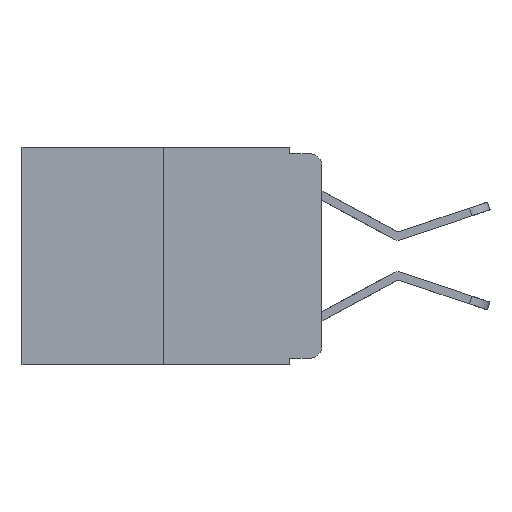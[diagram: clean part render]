
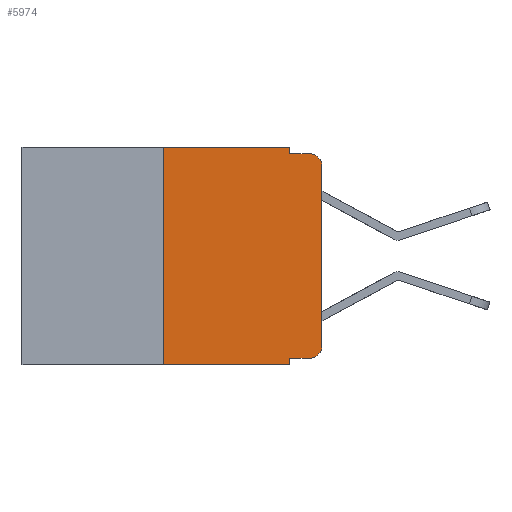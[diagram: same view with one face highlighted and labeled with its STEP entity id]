
A CAD part, left-side view. The second image highlights one B-rep face of the part: STEP entity #5974.
In plain terms, the highlighted planar face has unit normal (-1, 0, 0).
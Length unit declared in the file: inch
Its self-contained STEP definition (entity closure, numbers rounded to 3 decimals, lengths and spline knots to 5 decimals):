
#44 = CARTESIAN_POINT ( 'NONE',  ( 0., 0., 0. ) ) ;
#95 = CARTESIAN_POINT ( 'NONE',  ( 0., 0.473, 0. ) ) ;
#278 = LINE ( 'NONE', #5480, #4809 ) ;
#353 = EDGE_CURVE ( 'NONE', #7206, #18156, #7311, .T. ) ;
#650 = VERTEX_POINT ( 'NONE', #5163 ) ;
#682 = EDGE_CURVE ( 'NONE', #650, #17576, #9665, .T. ) ;
#1302 = ORIENTED_EDGE ( 'NONE', *, *, #15574, .F. ) ;
#1369 = VECTOR ( 'NONE', #10219, 39.37008 ) ;
#1646 = VECTOR ( 'NONE', #16651, 39.37008 ) ;
#2016 = ORIENTED_EDGE ( 'NONE', *, *, #12888, .T. ) ;
#2082 = EDGE_CURVE ( 'NONE', #650, #7614, #5396, .T. ) ;
#2386 = CARTESIAN_POINT ( 'NONE',  ( 0., 0.051, -0.01 ) ) ;
#2446 = CARTESIAN_POINT ( 'NONE',  ( 0., 0.02, -0.313 ) ) ;
#2654 = CARTESIAN_POINT ( 'NONE',  ( 0., 0.051, 0. ) ) ;
#2693 = LINE ( 'NONE', #13224, #3640 ) ;
#2829 = VERTEX_POINT ( 'NONE', #16984 ) ;
#2839 = EDGE_CURVE ( 'NONE', #2829, #3998, #11771, .T. ) ;
#2913 = VECTOR ( 'NONE', #13555, 39.37008 ) ;
#2977 = PLANE ( 'NONE',  #3297 ) ;
#3297 = AXIS2_PLACEMENT_3D ( 'NONE', #11960, #4524, #14995 ) ;
#3496 = CARTESIAN_POINT ( 'NONE',  ( 0., 0.051, -0.01 ) ) ;
#3525 = CARTESIAN_POINT ( 'NONE',  ( 0., 0.02, -0.03 ) ) ;
#3640 = VECTOR ( 'NONE', #4261, 39.37008 ) ;
#3788 = EDGE_LOOP ( 'NONE', ( #2016, #6495, #4403, #1302, #18246, #19176, #9107, #13548, #14967, #11889 ) ) ;
#3901 = DIRECTION ( 'NONE',  ( 0., -1., 0. ) ) ;
#3963 = DIRECTION ( 'NONE',  ( 0., 0., -1. ) ) ;
#3998 = VERTEX_POINT ( 'NONE', #14030 ) ;
#4228 = CARTESIAN_POINT ( 'NONE',  ( 0., 0.051, -0.333 ) ) ;
#4261 = DIRECTION ( 'NONE',  ( 0., 0., 1. ) ) ;
#4403 = ORIENTED_EDGE ( 'NONE', *, *, #15913, .F. ) ;
#4524 = DIRECTION ( 'NONE',  ( 1., 0., 0. ) ) ;
#4539 = CARTESIAN_POINT ( 'NONE',  ( 0., 0.25, 0. ) ) ;
#4809 = VECTOR ( 'NONE', #3901, 39.37008 ) ;
#5002 = AXIS2_PLACEMENT_3D ( 'NONE', #2446, #12935, #3963 ) ;
#5021 = DIRECTION ( 'NONE',  ( 0., -1., 0. ) ) ;
#5050 = DIRECTION ( 'NONE',  ( 0., 0., -1. ) ) ;
#5163 = CARTESIAN_POINT ( 'NONE',  ( 0., 0.051, -0.333 ) ) ;
#5396 = LINE ( 'NONE', #4228, #1369 ) ;
#5480 = CARTESIAN_POINT ( 'NONE',  ( 0., 0.473, -0.343 ) ) ;
#5594 = FACE_OUTER_BOUND ( 'NONE', #3788, .T. ) ;
#5750 = VERTEX_POINT ( 'NONE', #11143 ) ;
#5974 = ADVANCED_FACE ( 'NONE', ( #5594 ), #2977, .F. ) ;
#6495 = ORIENTED_EDGE ( 'NONE', *, *, #2839, .T. ) ;
#7098 = CARTESIAN_POINT ( 'NONE',  ( 0., 0., -0.313 ) ) ;
#7158 = VECTOR ( 'NONE', #5021, 39.37008 ) ;
#7206 = VERTEX_POINT ( 'NONE', #4539 ) ;
#7215 = CARTESIAN_POINT ( 'NONE',  ( 0., 0.051, -0.343 ) ) ;
#7311 = LINE ( 'NONE', #95, #11314 ) ;
#7565 = VERTEX_POINT ( 'NONE', #2386 ) ;
#7614 = VERTEX_POINT ( 'NONE', #14528 ) ;
#8063 = VERTEX_POINT ( 'NONE', #7098 ) ;
#8958 = AXIS2_PLACEMENT_3D ( 'NONE', #3525, #14005, #5050 ) ;
#9107 = ORIENTED_EDGE ( 'NONE', *, *, #13288, .T. ) ;
#9665 = LINE ( 'NONE', #15567, #1646 ) ;
#10038 = CARTESIAN_POINT ( 'NONE',  ( 0., 0.051, 0. ) ) ;
#10219 = DIRECTION ( 'NONE',  ( 0., -1., 0. ) ) ;
#11143 = CARTESIAN_POINT ( 'NONE',  ( 0., 0.25, -0.343 ) ) ;
#11314 = VECTOR ( 'NONE', #19327, 39.37008 ) ;
#11623 = DIRECTION ( 'NONE',  ( 0., 0., -1. ) ) ;
#11771 = CIRCLE ( 'NONE', #8958, 0.02 ) ;
#11824 = LINE ( 'NONE', #44, #2913 ) ;
#11889 = ORIENTED_EDGE ( 'NONE', *, *, #13273, .T. ) ;
#11960 = CARTESIAN_POINT ( 'NONE',  ( 0., 0.473, 0. ) ) ;
#12718 = EDGE_CURVE ( 'NONE', #5750, #7206, #2693, .T. ) ;
#12759 = CIRCLE ( 'NONE', #5002, 0.02 ) ;
#12888 = EDGE_CURVE ( 'NONE', #8063, #2829, #11824, .T. ) ;
#12935 = DIRECTION ( 'NONE',  ( -1., 0., 0. ) ) ;
#13224 = CARTESIAN_POINT ( 'NONE',  ( 0., 0.25, 0. ) ) ;
#13273 = EDGE_CURVE ( 'NONE', #7614, #8063, #12759, .T. ) ;
#13288 = EDGE_CURVE ( 'NONE', #5750, #17576, #278, .T. ) ;
#13548 = ORIENTED_EDGE ( 'NONE', *, *, #682, .F. ) ;
#13555 = DIRECTION ( 'NONE',  ( 0., 0., 1. ) ) ;
#13740 = VECTOR ( 'NONE', #11623, 39.37008 ) ;
#14005 = DIRECTION ( 'NONE',  ( -1., 0., 0. ) ) ;
#14030 = CARTESIAN_POINT ( 'NONE',  ( 0., 0.02, -0.01 ) ) ;
#14205 = LINE ( 'NONE', #2654, #13740 ) ;
#14528 = CARTESIAN_POINT ( 'NONE',  ( 0., 0.02, -0.333 ) ) ;
#14967 = ORIENTED_EDGE ( 'NONE', *, *, #2082, .T. ) ;
#14995 = DIRECTION ( 'NONE',  ( 0., 0., -1. ) ) ;
#15567 = CARTESIAN_POINT ( 'NONE',  ( 0., 0.051, 0. ) ) ;
#15574 = EDGE_CURVE ( 'NONE', #18156, #7565, #14205, .T. ) ;
#15913 = EDGE_CURVE ( 'NONE', #7565, #3998, #19131, .T. ) ;
#16651 = DIRECTION ( 'NONE',  ( 0., 0., -1. ) ) ;
#16984 = CARTESIAN_POINT ( 'NONE',  ( 0., 0., -0.03 ) ) ;
#17576 = VERTEX_POINT ( 'NONE', #7215 ) ;
#18156 = VERTEX_POINT ( 'NONE', #10038 ) ;
#18246 = ORIENTED_EDGE ( 'NONE', *, *, #353, .F. ) ;
#19131 = LINE ( 'NONE', #3496, #7158 ) ;
#19176 = ORIENTED_EDGE ( 'NONE', *, *, #12718, .F. ) ;
#19327 = DIRECTION ( 'NONE',  ( 0., -1., 0. ) ) ;
